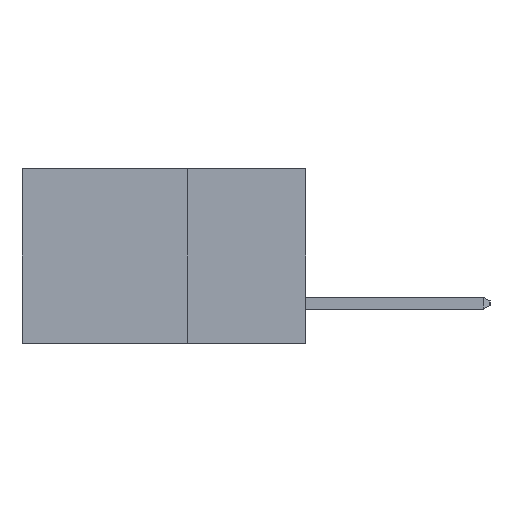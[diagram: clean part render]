
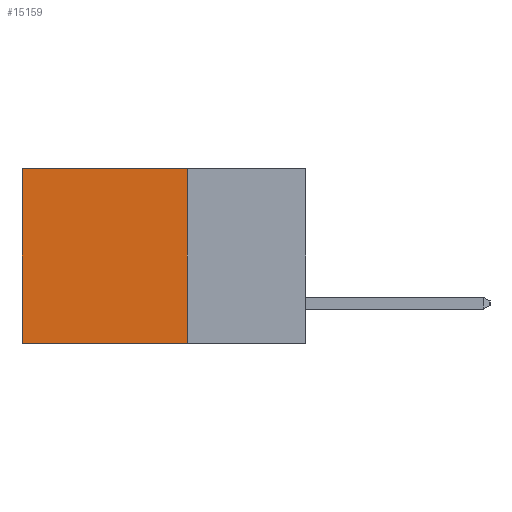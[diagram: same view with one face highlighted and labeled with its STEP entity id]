
A CAD part, left-side view. The second image highlights one B-rep face of the part: STEP entity #15159.
In plain terms, the highlighted planar face has unit normal (-1, 0, 0).
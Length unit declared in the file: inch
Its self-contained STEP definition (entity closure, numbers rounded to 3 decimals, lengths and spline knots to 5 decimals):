
#122 = ORIENTED_EDGE ( 'NONE', *, *, #14152, .T. ) ;
#505 = LINE ( 'NONE', #11607, #10975 ) ;
#565 = CARTESIAN_POINT ( 'NONE',  ( 0.298, 0.25, -0.37 ) ) ;
#1646 = ORIENTED_EDGE ( 'NONE', *, *, #13803, .F. ) ;
#2012 = DIRECTION ( 'NONE',  ( 0., 1., 0. ) ) ;
#3674 = EDGE_CURVE ( 'NONE', #3959, #8842, #8759, .T. ) ;
#3959 = VERTEX_POINT ( 'NONE', #7017 ) ;
#4533 = VECTOR ( 'NONE', #16489, 39.37008 ) ;
#4584 = CARTESIAN_POINT ( 'NONE',  ( 0.298, 0.25, -0.37 ) ) ;
#5575 = EDGE_CURVE ( 'NONE', #3959, #9953, #12671, .T. ) ;
#6198 = ORIENTED_EDGE ( 'NONE', *, *, #5575, .T. ) ;
#6720 = CARTESIAN_POINT ( 'NONE',  ( 0.298, 0.25, 0. ) ) ;
#7017 = CARTESIAN_POINT ( 'NONE',  ( 0.298, 0.25, 0. ) ) ;
#8161 = DIRECTION ( 'NONE',  ( 1., 0., 0. ) ) ;
#8759 = LINE ( 'NONE', #16548, #4533 ) ;
#8842 = VERTEX_POINT ( 'NONE', #4584 ) ;
#9158 = CARTESIAN_POINT ( 'NONE',  ( 0.298, 0.25, 0. ) ) ;
#9649 = VECTOR ( 'NONE', #2012, 39.37008 ) ;
#9953 = VERTEX_POINT ( 'NONE', #16316 ) ;
#10089 = LINE ( 'NONE', #565, #9649 ) ;
#10592 = DIRECTION ( 'NONE',  ( 0., 1., 0. ) ) ;
#10975 = VECTOR ( 'NONE', #13007, 39.37008 ) ;
#10984 = CARTESIAN_POINT ( 'NONE',  ( 0.298, 0.6, -0.37 ) ) ;
#11266 = EDGE_LOOP ( 'NONE', ( #122, #1646, #17966, #6198 ) ) ;
#11607 = CARTESIAN_POINT ( 'NONE',  ( 0.298, 0.6, 0. ) ) ;
#12671 = LINE ( 'NONE', #9158, #15972 ) ;
#13007 = DIRECTION ( 'NONE',  ( 0., 0., -1. ) ) ;
#13239 = FACE_OUTER_BOUND ( 'NONE', #11266, .T. ) ;
#13803 = EDGE_CURVE ( 'NONE', #8842, #17675, #10089, .T. ) ;
#14152 = EDGE_CURVE ( 'NONE', #9953, #17675, #505, .T. ) ;
#14494 = AXIS2_PLACEMENT_3D ( 'NONE', #6720, #8161, #17989 ) ;
#15159 = ADVANCED_FACE ( 'NONE', ( #13239 ), #16602, .F. ) ;
#15972 = VECTOR ( 'NONE', #10592, 39.37008 ) ;
#16316 = CARTESIAN_POINT ( 'NONE',  ( 0.298, 0.6, 0. ) ) ;
#16489 = DIRECTION ( 'NONE',  ( 0., 0., -1. ) ) ;
#16548 = CARTESIAN_POINT ( 'NONE',  ( 0.298, 0.25, 0. ) ) ;
#16602 = PLANE ( 'NONE',  #14494 ) ;
#17675 = VERTEX_POINT ( 'NONE', #10984 ) ;
#17966 = ORIENTED_EDGE ( 'NONE', *, *, #3674, .F. ) ;
#17989 = DIRECTION ( 'NONE',  ( 0., 0., -1. ) ) ;
